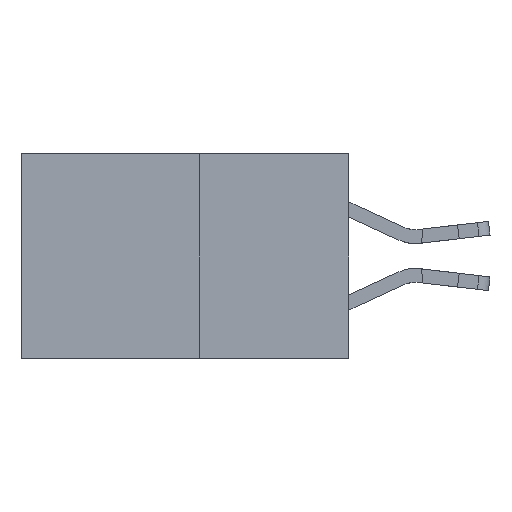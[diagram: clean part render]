
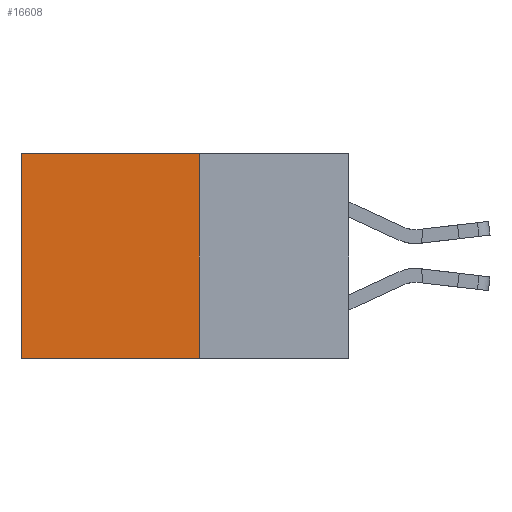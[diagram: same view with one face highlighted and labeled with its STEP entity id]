
A CAD part, left-side view. The second image highlights one B-rep face of the part: STEP entity #16608.
In plain terms, the highlighted planar face has unit normal (-1, 0, 0).
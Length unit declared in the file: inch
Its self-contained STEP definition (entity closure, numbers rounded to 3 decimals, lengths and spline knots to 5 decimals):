
#306 = EDGE_CURVE ( 'NONE', #8857, #20120, #11394, .T. ) ;
#1181 = VECTOR ( 'NONE', #10048, 39.37008 ) ;
#1400 = LINE ( 'NONE', #17279, #10137 ) ;
#1783 = EDGE_CURVE ( 'NONE', #20120, #11198, #5280, .T. ) ;
#2648 = VECTOR ( 'NONE', #20598, 39.37008 ) ;
#3808 = ORIENTED_EDGE ( 'NONE', *, *, #9739, .T. ) ;
#4108 = CARTESIAN_POINT ( 'NONE',  ( 0.277, 0.27, -0.37 ) ) ;
#5142 = ORIENTED_EDGE ( 'NONE', *, *, #1783, .F. ) ;
#5280 = LINE ( 'NONE', #9450, #1181 ) ;
#7471 = VECTOR ( 'NONE', #12997, 39.37008 ) ;
#7868 = DIRECTION ( 'NONE',  ( 1., 0., 0. ) ) ;
#8676 = ORIENTED_EDGE ( 'NONE', *, *, #8853, .T. ) ;
#8853 = EDGE_CURVE ( 'NONE', #14321, #11198, #16655, .T. ) ;
#8857 = VERTEX_POINT ( 'NONE', #13071 ) ;
#9450 = CARTESIAN_POINT ( 'NONE',  ( 0.277, 0.27, -0.37 ) ) ;
#9489 = CARTESIAN_POINT ( 'NONE',  ( 0.277, 0.59, -0.37 ) ) ;
#9739 = EDGE_CURVE ( 'NONE', #8857, #14321, #1400, .T. ) ;
#10048 = DIRECTION ( 'NONE',  ( 0., 1., 0. ) ) ;
#10137 = VECTOR ( 'NONE', #18961, 39.37008 ) ;
#10821 = ORIENTED_EDGE ( 'NONE', *, *, #306, .F. ) ;
#11198 = VERTEX_POINT ( 'NONE', #17172 ) ;
#11394 = LINE ( 'NONE', #4108, #2648 ) ;
#11570 = FACE_OUTER_BOUND ( 'NONE', #13973, .T. ) ;
#12660 = CARTESIAN_POINT ( 'NONE',  ( 0.277, 0.27, -0.37 ) ) ;
#12753 = AXIS2_PLACEMENT_3D ( 'NONE', #18145, #7868, #19841 ) ;
#12997 = DIRECTION ( 'NONE',  ( 0., 0., -1. ) ) ;
#13071 = CARTESIAN_POINT ( 'NONE',  ( 0.277, 0.27, 0. ) ) ;
#13973 = EDGE_LOOP ( 'NONE', ( #8676, #5142, #10821, #3808 ) ) ;
#14321 = VERTEX_POINT ( 'NONE', #15084 ) ;
#15084 = CARTESIAN_POINT ( 'NONE',  ( 0.277, 0.59, 0. ) ) ;
#16608 = ADVANCED_FACE ( 'NONE', ( #11570 ), #21439, .F. ) ;
#16655 = LINE ( 'NONE', #9489, #7471 ) ;
#17172 = CARTESIAN_POINT ( 'NONE',  ( 0.277, 0.59, -0.37 ) ) ;
#17279 = CARTESIAN_POINT ( 'NONE',  ( 0.277, 0.27, 0. ) ) ;
#18145 = CARTESIAN_POINT ( 'NONE',  ( 0.277, 0.27, -0.37 ) ) ;
#18961 = DIRECTION ( 'NONE',  ( 0., 1., 0. ) ) ;
#19841 = DIRECTION ( 'NONE',  ( 0., 0., -1. ) ) ;
#20120 = VERTEX_POINT ( 'NONE', #12660 ) ;
#20598 = DIRECTION ( 'NONE',  ( 0., 0., -1. ) ) ;
#21439 = PLANE ( 'NONE',  #12753 ) ;
